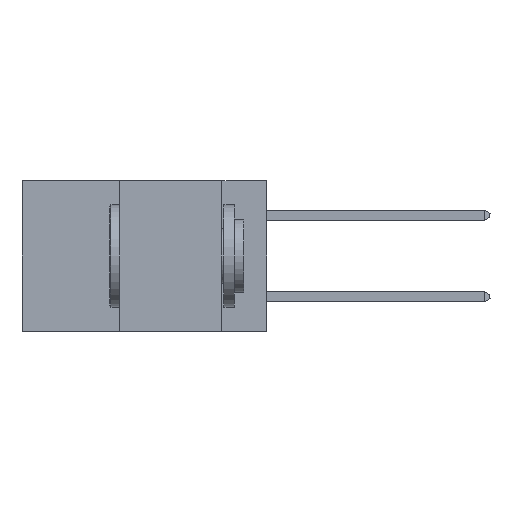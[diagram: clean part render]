
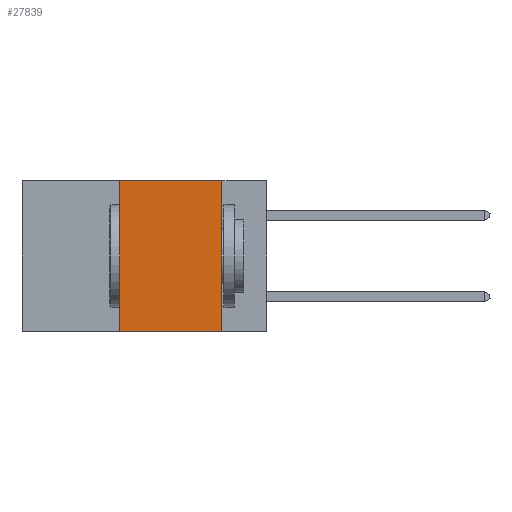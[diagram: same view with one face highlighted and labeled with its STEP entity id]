
A CAD part, left-side view. The second image highlights one B-rep face of the part: STEP entity #27839.
In plain terms, the highlighted planar face has unit normal (-1, 0, 0).
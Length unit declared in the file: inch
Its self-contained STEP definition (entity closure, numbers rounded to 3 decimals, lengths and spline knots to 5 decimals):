
#2752 = CARTESIAN_POINT ( 'NONE',  ( 0., 0.6, 0. ) ) ;
#3257 = AXIS2_PLACEMENT_3D ( 'NONE', #33645, #36493, #19291 ) ;
#4792 = VERTEX_POINT ( 'NONE', #33531 ) ;
#4911 = EDGE_CURVE ( 'NONE', #4792, #14033, #14031, .T. ) ;
#5451 = CARTESIAN_POINT ( 'NONE',  ( 0., 0.36, 0. ) ) ;
#6156 = VECTOR ( 'NONE', #22980, 39.37008 ) ;
#6194 = CARTESIAN_POINT ( 'NONE',  ( 0., 0.36, 0. ) ) ;
#6332 = VECTOR ( 'NONE', #33250, 39.37008 ) ;
#6515 = DIRECTION ( 'NONE',  ( 0., -1., 0. ) ) ;
#8309 = CARTESIAN_POINT ( 'NONE',  ( 0., 0.11, 0. ) ) ;
#8939 = ORIENTED_EDGE ( 'NONE', *, *, #32029, .F. ) ;
#9859 = ORIENTED_EDGE ( 'NONE', *, *, #14790, .T. ) ;
#11299 = DIRECTION ( 'NONE',  ( 0., 0., -1. ) ) ;
#12336 = CARTESIAN_POINT ( 'NONE',  ( 0., 0.6, -0.37 ) ) ;
#13898 = EDGE_LOOP ( 'NONE', ( #36988, #8939, #16777, #9859 ) ) ;
#14031 = LINE ( 'NONE', #5451, #6156 ) ;
#14033 = VERTEX_POINT ( 'NONE', #6194 ) ;
#14790 = EDGE_CURVE ( 'NONE', #4792, #29033, #23697, .T. ) ;
#15982 = VECTOR ( 'NONE', #6515, 39.37008 ) ;
#16777 = ORIENTED_EDGE ( 'NONE', *, *, #4911, .F. ) ;
#18582 = CARTESIAN_POINT ( 'NONE',  ( 0., 0.11, -0.37 ) ) ;
#19291 = DIRECTION ( 'NONE',  ( 0., 0., -1. ) ) ;
#19809 = FACE_OUTER_BOUND ( 'NONE', #13898, .T. ) ;
#22719 = LINE ( 'NONE', #8309, #35299 ) ;
#22980 = DIRECTION ( 'NONE',  ( 0., 0., 1. ) ) ;
#23697 = LINE ( 'NONE', #12336, #15982 ) ;
#24014 = VERTEX_POINT ( 'NONE', #36392 ) ;
#27839 = ADVANCED_FACE ( 'NONE', ( #19809 ), #30777, .F. ) ;
#29033 = VERTEX_POINT ( 'NONE', #18582 ) ;
#29547 = LINE ( 'NONE', #2752, #6332 ) ;
#30777 = PLANE ( 'NONE',  #3257 ) ;
#32029 = EDGE_CURVE ( 'NONE', #14033, #24014, #29547, .T. ) ;
#32949 = EDGE_CURVE ( 'NONE', #24014, #29033, #22719, .T. ) ;
#33250 = DIRECTION ( 'NONE',  ( 0., -1., 0. ) ) ;
#33531 = CARTESIAN_POINT ( 'NONE',  ( 0., 0.36, -0.37 ) ) ;
#33645 = CARTESIAN_POINT ( 'NONE',  ( 0., 0.6, 0. ) ) ;
#35299 = VECTOR ( 'NONE', #11299, 39.37008 ) ;
#36392 = CARTESIAN_POINT ( 'NONE',  ( 0., 0.11, 0. ) ) ;
#36493 = DIRECTION ( 'NONE',  ( 1., 0., 0. ) ) ;
#36988 = ORIENTED_EDGE ( 'NONE', *, *, #32949, .F. ) ;
